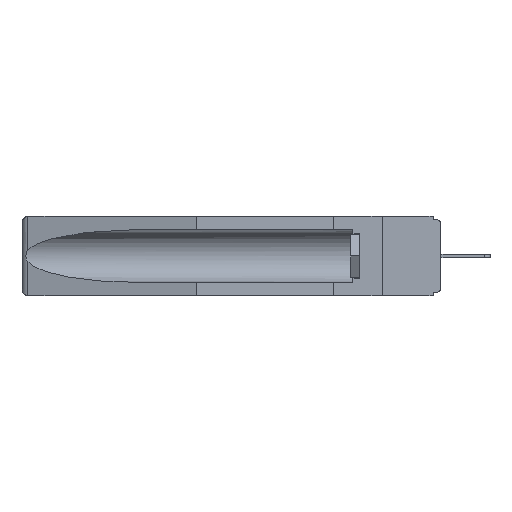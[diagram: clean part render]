
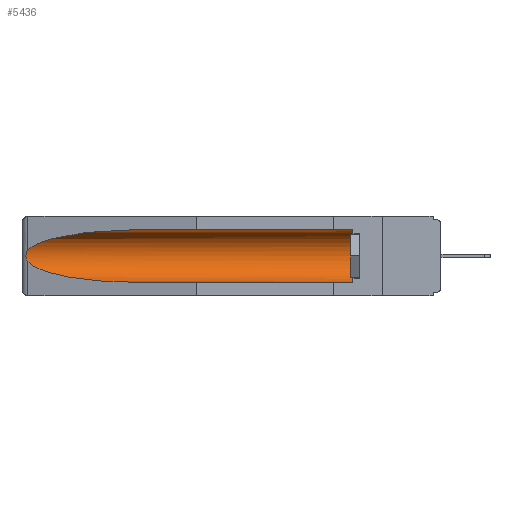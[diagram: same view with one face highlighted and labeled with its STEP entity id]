
A CAD part, left-side view. The second image highlights one B-rep face of the part: STEP entity #5436.
In plain terms, the highlighted cylindrical face has radius 2.857 mm (diameter 5.715 mm), a partial arc.
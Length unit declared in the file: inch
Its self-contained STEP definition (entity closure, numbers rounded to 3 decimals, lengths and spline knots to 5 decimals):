
#221 = CARTESIAN_POINT ( 'NONE',  ( 0.26537, 1.52718, -0.14972 ) ) ;
#259 = VERTEX_POINT ( 'NONE', #12153 ) ;
#426 = EDGE_CURVE ( 'NONE', #18403, #1942, #18247, .T. ) ;
#614 = CARTESIAN_POINT ( 'NONE',  ( 0.155, 1.07973, -0.059 ) ) ;
#942 = DIRECTION ( 'NONE',  ( 0., 1., 0. ) ) ;
#1147 = DIRECTION ( 'NONE',  ( 0., 0., 1. ) ) ;
#1738 = EDGE_CURVE ( 'NONE', #18403, #259, #4179, .T. ) ;
#1942 = VERTEX_POINT ( 'NONE', #9317 ) ;
#2209 = B_SPLINE_CURVE_WITH_KNOTS ( 'NONE', 3,
 ( #10790, #9283, #15417, #8271, #8568, #15995, #12865, #8458, #5433, #9867 ),
 .UNSPECIFIED., .F., .F.,
 ( 4, 2, 2, 2, 4 ),
 ( 0., 0.00029, 0.00058, 0.00087, 0.00117 ),
 .UNSPECIFIED. ) ;
#2282 = ORIENTED_EDGE ( 'NONE', *, *, #426, .T. ) ;
#3123 =( BOUNDED_CURVE ( )  B_SPLINE_CURVE ( 3, ( #11082, #18721, #5141, #221 ),
 .UNSPECIFIED., .F., .F. ) 
 B_SPLINE_CURVE_WITH_KNOTS ( ( 4, 4 ),
 ( 4.71239, 6.08839 ),
 .UNSPECIFIED. ) 
 CURVE ( )  GEOMETRIC_REPRESENTATION_ITEM ( )  RATIONAL_B_SPLINE_CURVE ( ( 1., 0.848, 0.848, 1. ) ) 
 REPRESENTATION_ITEM ( '' )  );
#3574 = DIRECTION ( 'NONE',  ( 0., -1., 0. ) ) ;
#3822 = VECTOR ( 'NONE', #12959, 39.37008 ) ;
#4179 = LINE ( 'NONE', #15984, #3822 ) ;
#4304 =( BOUNDED_CURVE ( )  B_SPLINE_CURVE ( 3, ( #18802, #10950, #5028, #5120 ),
 .UNSPECIFIED., .F., .F. ) 
 B_SPLINE_CURVE_WITH_KNOTS ( ( 4, 4 ),
 ( 0.1948, 1.5708 ),
 .UNSPECIFIED. ) 
 CURVE ( )  GEOMETRIC_REPRESENTATION_ITEM ( )  RATIONAL_B_SPLINE_CURVE ( ( 1., 0.848, 0.848, 1. ) ) 
 REPRESENTATION_ITEM ( '' )  );
#4762 = AXIS2_PLACEMENT_3D ( 'NONE', #14246, #3574, #18590 ) ;
#5002 = CARTESIAN_POINT ( 'NONE',  ( 0.155, 0.126, -0.284 ) ) ;
#5028 = CARTESIAN_POINT ( 'NONE',  ( 0.21114, 1.30732, -0.284 ) ) ;
#5120 = CARTESIAN_POINT ( 'NONE',  ( 0.155, 1.07973, -0.284 ) ) ;
#5141 = CARTESIAN_POINT ( 'NONE',  ( 0.25451, 1.48313, -0.09465 ) ) ;
#5433 = CARTESIAN_POINT ( 'NONE',  ( 0.26597, 1.5296, -0.19026 ) ) ;
#5436 = ADVANCED_FACE ( 'NONE', ( #9836 ), #14733, .F. ) ;
#5756 = ORIENTED_EDGE ( 'NONE', *, *, #11506, .T. ) ;
#6622 = CARTESIAN_POINT ( 'NONE',  ( 0.155, -0.30754, -0.1715 ) ) ;
#8271 = CARTESIAN_POINT ( 'NONE',  ( 0.2673, 1.5327, -0.16383 ) ) ;
#8458 = CARTESIAN_POINT ( 'NONE',  ( 0.26655, 1.53094, -0.18657 ) ) ;
#8568 = CARTESIAN_POINT ( 'NONE',  ( 0.2675, 1.53308, -0.16763 ) ) ;
#8678 = EDGE_LOOP ( 'NONE', ( #5756, #16972, #16728, #11600, #2282, #8931 ) ) ;
#8931 = ORIENTED_EDGE ( 'NONE', *, *, #13006, .T. ) ;
#8943 = LINE ( 'NONE', #13549, #10160 ) ;
#9088 = EDGE_CURVE ( 'NONE', #15436, #15931, #2209, .T. ) ;
#9283 = CARTESIAN_POINT ( 'NONE',  ( 0.26597, 1.52961, -0.15275 ) ) ;
#9317 = CARTESIAN_POINT ( 'NONE',  ( 0.155, 0.126, -0.059 ) ) ;
#9836 = FACE_OUTER_BOUND ( 'NONE', #8678, .T. ) ;
#9867 = CARTESIAN_POINT ( 'NONE',  ( 0.26537, 1.52718, -0.19328 ) ) ;
#10160 = VECTOR ( 'NONE', #19587, 39.37008 ) ;
#10790 = CARTESIAN_POINT ( 'NONE',  ( 0.26537, 1.52718, -0.14972 ) ) ;
#10950 = CARTESIAN_POINT ( 'NONE',  ( 0.25451, 1.48313, -0.24835 ) ) ;
#11082 = CARTESIAN_POINT ( 'NONE',  ( 0.155, 1.07973, -0.059 ) ) ;
#11506 = EDGE_CURVE ( 'NONE', #14084, #15436, #3123, .T. ) ;
#11600 = ORIENTED_EDGE ( 'NONE', *, *, #1738, .F. ) ;
#11957 = EDGE_CURVE ( 'NONE', #15931, #259, #4304, .T. ) ;
#12153 = CARTESIAN_POINT ( 'NONE',  ( 0.155, 1.07973, -0.284 ) ) ;
#12865 = CARTESIAN_POINT ( 'NONE',  ( 0.2673, 1.53269, -0.17917 ) ) ;
#12959 = DIRECTION ( 'NONE',  ( 0., 1., 0. ) ) ;
#13006 = EDGE_CURVE ( 'NONE', #1942, #14084, #8943, .T. ) ;
#13549 = CARTESIAN_POINT ( 'NONE',  ( 0.155, -0.30754, -0.059 ) ) ;
#14084 = VERTEX_POINT ( 'NONE', #614 ) ;
#14246 = CARTESIAN_POINT ( 'NONE',  ( 0.155, 0.126, -0.1715 ) ) ;
#14409 = CARTESIAN_POINT ( 'NONE',  ( 0.26537, 1.52718, -0.14972 ) ) ;
#14475 = CARTESIAN_POINT ( 'NONE',  ( 0.26537, 1.52718, -0.19328 ) ) ;
#14733 = CYLINDRICAL_SURFACE ( 'NONE', #19380, 0.1125 ) ;
#15417 = CARTESIAN_POINT ( 'NONE',  ( 0.26654, 1.53092, -0.15636 ) ) ;
#15436 = VERTEX_POINT ( 'NONE', #14409 ) ;
#15931 = VERTEX_POINT ( 'NONE', #14475 ) ;
#15984 = CARTESIAN_POINT ( 'NONE',  ( 0.155, -0.30754, -0.284 ) ) ;
#15995 = CARTESIAN_POINT ( 'NONE',  ( 0.2675, 1.53308, -0.17534 ) ) ;
#16728 = ORIENTED_EDGE ( 'NONE', *, *, #11957, .T. ) ;
#16972 = ORIENTED_EDGE ( 'NONE', *, *, #9088, .T. ) ;
#18247 = CIRCLE ( 'NONE', #4762, 0.1125 ) ;
#18403 = VERTEX_POINT ( 'NONE', #5002 ) ;
#18590 = DIRECTION ( 'NONE',  ( 0., 0., 1. ) ) ;
#18721 = CARTESIAN_POINT ( 'NONE',  ( 0.21114, 1.30732, -0.059 ) ) ;
#18802 = CARTESIAN_POINT ( 'NONE',  ( 0.26537, 1.52718, -0.19328 ) ) ;
#19380 = AXIS2_PLACEMENT_3D ( 'NONE', #6622, #942, #1147 ) ;
#19587 = DIRECTION ( 'NONE',  ( 0., 1., 0. ) ) ;
